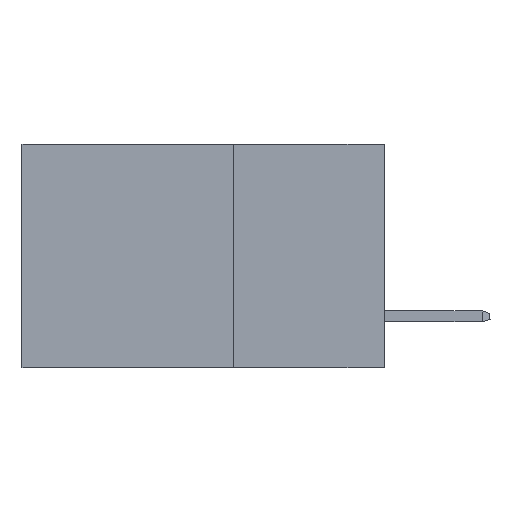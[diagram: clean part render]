
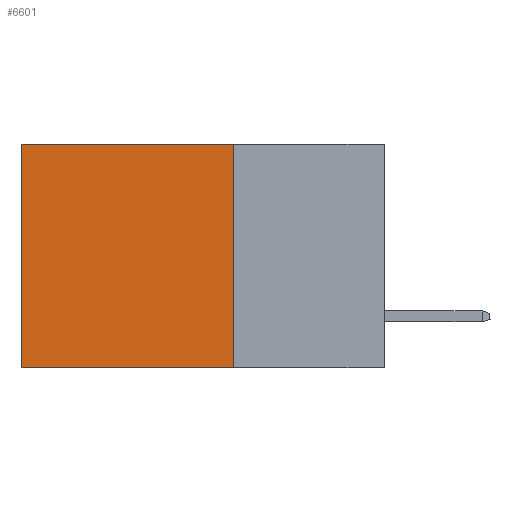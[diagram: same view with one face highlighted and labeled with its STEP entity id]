
A CAD part, left-side view. The second image highlights one B-rep face of the part: STEP entity #6601.
In plain terms, the highlighted planar face has unit normal (-1, 0, 0).
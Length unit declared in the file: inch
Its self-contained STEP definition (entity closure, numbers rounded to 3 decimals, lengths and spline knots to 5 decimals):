
#1139 = VECTOR ( 'NONE', #4052, 39.37008 ) ;
#2020 = CARTESIAN_POINT ( 'NONE',  ( 0.298, 0.25, 0. ) ) ;
#3278 = EDGE_LOOP ( 'NONE', ( #14030, #12420, #15497, #15003 ) ) ;
#3513 = DIRECTION ( 'NONE',  ( 0., 0., -1. ) ) ;
#3733 = DIRECTION ( 'NONE',  ( 1., 0., 0. ) ) ;
#3851 = PLANE ( 'NONE',  #5987 ) ;
#4052 = DIRECTION ( 'NONE',  ( 0., 1., 0. ) ) ;
#4328 = CARTESIAN_POINT ( 'NONE',  ( 0.298, 0.25, 0. ) ) ;
#4448 = VERTEX_POINT ( 'NONE', #14146 ) ;
#5039 = CARTESIAN_POINT ( 'NONE',  ( 0.298, 0.25, 0. ) ) ;
#5593 = DIRECTION ( 'NONE',  ( 0., 0., -1. ) ) ;
#5787 = VECTOR ( 'NONE', #3513, 39.37008 ) ;
#5987 = AXIS2_PLACEMENT_3D ( 'NONE', #9017, #3733, #6309 ) ;
#6192 = LINE ( 'NONE', #12505, #5787 ) ;
#6309 = DIRECTION ( 'NONE',  ( 0., 0., -1. ) ) ;
#6601 = ADVANCED_FACE ( 'NONE', ( #11838 ), #3851, .F. ) ;
#7452 = VERTEX_POINT ( 'NONE', #9614 ) ;
#7673 = LINE ( 'NONE', #12869, #1139 ) ;
#7831 = DIRECTION ( 'NONE',  ( 0., 1., 0. ) ) ;
#9017 = CARTESIAN_POINT ( 'NONE',  ( 0.298, 0.25, 0. ) ) ;
#9087 = VECTOR ( 'NONE', #7831, 39.37008 ) ;
#9614 = CARTESIAN_POINT ( 'NONE',  ( 0.298, 0.6, -0.37 ) ) ;
#9991 = VECTOR ( 'NONE', #5593, 39.37008 ) ;
#10995 = EDGE_CURVE ( 'NONE', #16460, #7452, #7673, .T. ) ;
#11696 = VERTEX_POINT ( 'NONE', #2020 ) ;
#11838 = FACE_OUTER_BOUND ( 'NONE', #3278, .T. ) ;
#12420 = ORIENTED_EDGE ( 'NONE', *, *, #10995, .F. ) ;
#12505 = CARTESIAN_POINT ( 'NONE',  ( 0.298, 0.6, 0. ) ) ;
#12869 = CARTESIAN_POINT ( 'NONE',  ( 0.298, 0.25, -0.37 ) ) ;
#13413 = LINE ( 'NONE', #4328, #9991 ) ;
#13569 = CARTESIAN_POINT ( 'NONE',  ( 0.298, 0.25, -0.37 ) ) ;
#13718 = LINE ( 'NONE', #5039, #9087 ) ;
#13816 = EDGE_CURVE ( 'NONE', #11696, #16460, #13413, .T. ) ;
#14030 = ORIENTED_EDGE ( 'NONE', *, *, #14770, .T. ) ;
#14146 = CARTESIAN_POINT ( 'NONE',  ( 0.298, 0.6, 0. ) ) ;
#14770 = EDGE_CURVE ( 'NONE', #4448, #7452, #6192, .T. ) ;
#15003 = ORIENTED_EDGE ( 'NONE', *, *, #16447, .T. ) ;
#15497 = ORIENTED_EDGE ( 'NONE', *, *, #13816, .F. ) ;
#16447 = EDGE_CURVE ( 'NONE', #11696, #4448, #13718, .T. ) ;
#16460 = VERTEX_POINT ( 'NONE', #13569 ) ;
